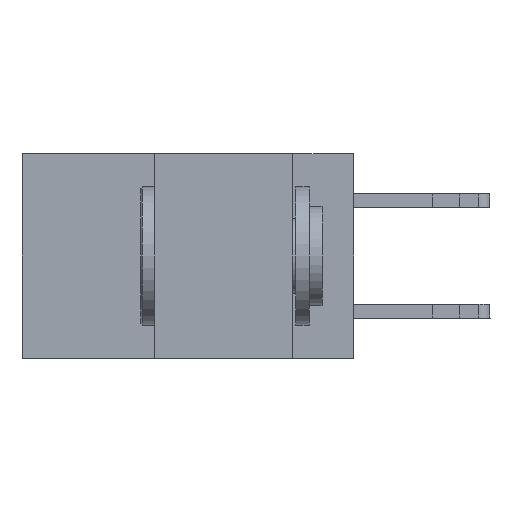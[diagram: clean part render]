
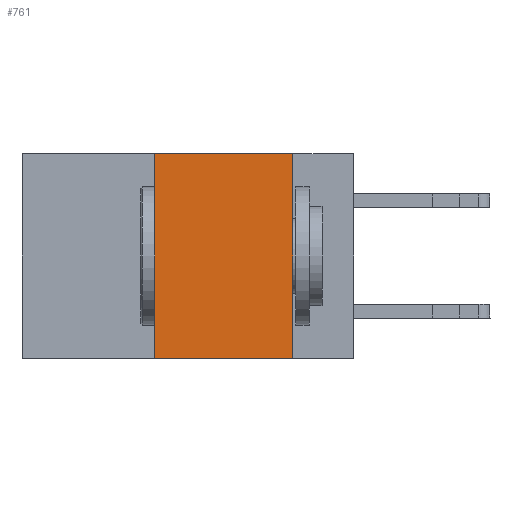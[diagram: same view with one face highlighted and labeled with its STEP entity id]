
A CAD part, left-side view. The second image highlights one B-rep face of the part: STEP entity #761.
In plain terms, the highlighted planar face has unit normal (-1, 0, 0).
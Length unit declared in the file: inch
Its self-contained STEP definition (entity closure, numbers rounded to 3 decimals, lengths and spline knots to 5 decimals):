
#585 = CARTESIAN_POINT ( 'NONE',  ( 0., 0.6, -0.37 ) ) ;
#761 = ADVANCED_FACE ( 'NONE', ( #9270 ), #4855, .F. ) ;
#1509 = EDGE_LOOP ( 'NONE', ( #19783, #9436, #19026, #27189 ) ) ;
#2288 = LINE ( 'NONE', #13635, #4795 ) ;
#3412 = VECTOR ( 'NONE', #25566, 39.37008 ) ;
#3813 = CARTESIAN_POINT ( 'NONE',  ( 0., 0.11, -0.37 ) ) ;
#4038 = CARTESIAN_POINT ( 'NONE',  ( 0., 0.11, 0. ) ) ;
#4624 = CARTESIAN_POINT ( 'NONE',  ( 0., 0.36, 0. ) ) ;
#4795 = VECTOR ( 'NONE', #25056, 39.37008 ) ;
#4855 = PLANE ( 'NONE',  #10693 ) ;
#7100 = EDGE_CURVE ( 'NONE', #21270, #8428, #29726, .T. ) ;
#7488 = LINE ( 'NONE', #29759, #10386 ) ;
#8428 = VERTEX_POINT ( 'NONE', #3813 ) ;
#9270 = FACE_OUTER_BOUND ( 'NONE', #1509, .T. ) ;
#9436 = ORIENTED_EDGE ( 'NONE', *, *, #25800, .F. ) ;
#10002 = VECTOR ( 'NONE', #22639, 39.37008 ) ;
#10386 = VECTOR ( 'NONE', #23687, 39.37008 ) ;
#10693 = AXIS2_PLACEMENT_3D ( 'NONE', #22767, #15944, #18244 ) ;
#12088 = EDGE_CURVE ( 'NONE', #21270, #24278, #19327, .T. ) ;
#13635 = CARTESIAN_POINT ( 'NONE',  ( 0., 0.11, 0. ) ) ;
#14908 = CARTESIAN_POINT ( 'NONE',  ( 0., 0.36, -0.37 ) ) ;
#15466 = VERTEX_POINT ( 'NONE', #4038 ) ;
#15944 = DIRECTION ( 'NONE',  ( 1., 0., 0. ) ) ;
#18244 = DIRECTION ( 'NONE',  ( 0., 0., -1. ) ) ;
#19026 = ORIENTED_EDGE ( 'NONE', *, *, #12088, .F. ) ;
#19327 = LINE ( 'NONE', #4624, #10002 ) ;
#19783 = ORIENTED_EDGE ( 'NONE', *, *, #22789, .F. ) ;
#21270 = VERTEX_POINT ( 'NONE', #14908 ) ;
#22639 = DIRECTION ( 'NONE',  ( 0., 0., 1. ) ) ;
#22767 = CARTESIAN_POINT ( 'NONE',  ( 0., 0.6, 0. ) ) ;
#22789 = EDGE_CURVE ( 'NONE', #15466, #8428, #2288, .T. ) ;
#23687 = DIRECTION ( 'NONE',  ( 0., -1., 0. ) ) ;
#24278 = VERTEX_POINT ( 'NONE', #24721 ) ;
#24721 = CARTESIAN_POINT ( 'NONE',  ( 0., 0.36, 0. ) ) ;
#25056 = DIRECTION ( 'NONE',  ( 0., 0., -1. ) ) ;
#25566 = DIRECTION ( 'NONE',  ( 0., -1., 0. ) ) ;
#25800 = EDGE_CURVE ( 'NONE', #24278, #15466, #7488, .T. ) ;
#27189 = ORIENTED_EDGE ( 'NONE', *, *, #7100, .T. ) ;
#29726 = LINE ( 'NONE', #585, #3412 ) ;
#29759 = CARTESIAN_POINT ( 'NONE',  ( 0., 0.6, 0. ) ) ;
